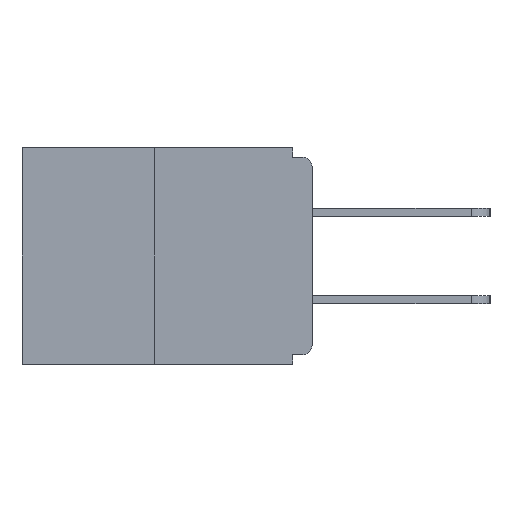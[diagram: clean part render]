
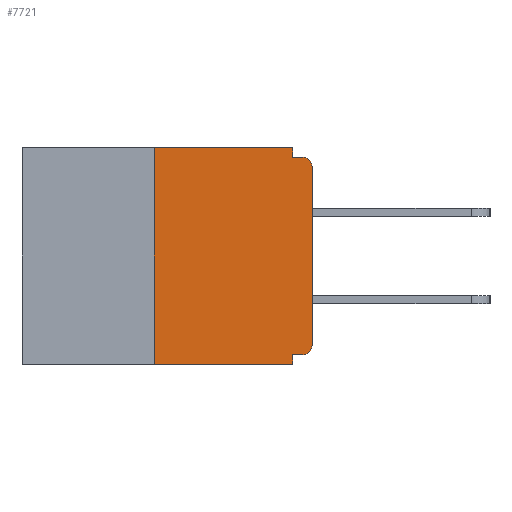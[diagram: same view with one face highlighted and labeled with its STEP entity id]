
A CAD part, left-side view. The second image highlights one B-rep face of the part: STEP entity #7721.
In plain terms, the highlighted planar face has unit normal (-1, 0, 0).
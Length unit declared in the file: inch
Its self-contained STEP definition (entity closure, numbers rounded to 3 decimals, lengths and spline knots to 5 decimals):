
#87 = CARTESIAN_POINT ( 'NONE',  ( 0., 0., -0.328 ) ) ;
#189 = CARTESIAN_POINT ( 'NONE',  ( 0., 0., 0. ) ) ;
#218 = ORIENTED_EDGE ( 'NONE', *, *, #12338, .T. ) ;
#695 = DIRECTION ( 'NONE',  ( 1., 0., 0. ) ) ;
#977 = CARTESIAN_POINT ( 'NONE',  ( 0., 0.031, 0. ) ) ;
#1492 = AXIS2_PLACEMENT_3D ( 'NONE', #21524, #695, #2453 ) ;
#1851 = DIRECTION ( 'NONE',  ( 0., 0., -1. ) ) ;
#1972 = DIRECTION ( 'NONE',  ( 0., 0., -1. ) ) ;
#1976 = VECTOR ( 'NONE', #21056, 39.37008 ) ;
#2016 = CIRCLE ( 'NONE', #18868, 0.015 ) ;
#2453 = DIRECTION ( 'NONE',  ( 0., 0., -1. ) ) ;
#2522 = ORIENTED_EDGE ( 'NONE', *, *, #21135, .F. ) ;
#3196 = CARTESIAN_POINT ( 'NONE',  ( 0., 0., -0.03 ) ) ;
#3369 = CARTESIAN_POINT ( 'NONE',  ( 0., 0.25, -0.343 ) ) ;
#4028 = EDGE_CURVE ( 'NONE', #12439, #8589, #10432, .T. ) ;
#4132 = DIRECTION ( 'NONE',  ( 0., 1., 0. ) ) ;
#4145 = VECTOR ( 'NONE', #10643, 39.37008 ) ;
#4317 = LINE ( 'NONE', #5608, #10608 ) ;
#4392 = ORIENTED_EDGE ( 'NONE', *, *, #21631, .T. ) ;
#4713 = VECTOR ( 'NONE', #19308, 39.37008 ) ;
#4917 = CARTESIAN_POINT ( 'NONE',  ( 0., 0.031, -0.015 ) ) ;
#4936 = ORIENTED_EDGE ( 'NONE', *, *, #24566, .F. ) ;
#5274 = CARTESIAN_POINT ( 'NONE',  ( 0., 0.25, 0. ) ) ;
#5608 = CARTESIAN_POINT ( 'NONE',  ( 0., 0.46, -0.343 ) ) ;
#5776 = CARTESIAN_POINT ( 'NONE',  ( 0., 0.015, -0.328 ) ) ;
#5835 = LINE ( 'NONE', #24543, #6129 ) ;
#6129 = VECTOR ( 'NONE', #10863, 39.37008 ) ;
#6374 = ORIENTED_EDGE ( 'NONE', *, *, #9918, .T. ) ;
#6804 = CARTESIAN_POINT ( 'NONE',  ( 0., 0.031, -0.343 ) ) ;
#6998 = DIRECTION ( 'NONE',  ( -1., 0., 0. ) ) ;
#7721 = ADVANCED_FACE ( 'NONE', ( #10244 ), #21444, .F. ) ;
#7835 = EDGE_CURVE ( 'NONE', #17323, #21360, #9649, .T. ) ;
#8450 = CARTESIAN_POINT ( 'NONE',  ( 0., 0.015, -0.015 ) ) ;
#8589 = VERTEX_POINT ( 'NONE', #24589 ) ;
#8884 = VERTEX_POINT ( 'NONE', #5274 ) ;
#9649 = LINE ( 'NONE', #20256, #17403 ) ;
#9728 = VERTEX_POINT ( 'NONE', #977 ) ;
#9918 = EDGE_CURVE ( 'NONE', #16723, #21360, #11314, .T. ) ;
#10037 = LINE ( 'NONE', #12642, #1976 ) ;
#10227 = ORIENTED_EDGE ( 'NONE', *, *, #11829, .F. ) ;
#10244 = FACE_OUTER_BOUND ( 'NONE', #12458, .T. ) ;
#10353 = VERTEX_POINT ( 'NONE', #5776 ) ;
#10432 = LINE ( 'NONE', #6804, #4145 ) ;
#10608 = VECTOR ( 'NONE', #17289, 39.37008 ) ;
#10643 = DIRECTION ( 'NONE',  ( 0., 0., -1. ) ) ;
#10863 = DIRECTION ( 'NONE',  ( 0., -1., 0. ) ) ;
#11314 = CIRCLE ( 'NONE', #18311, 0.015 ) ;
#11829 = EDGE_CURVE ( 'NONE', #10353, #12439, #13964, .T. ) ;
#12338 = EDGE_CURVE ( 'NONE', #18425, #16723, #15742, .T. ) ;
#12439 = VERTEX_POINT ( 'NONE', #14061 ) ;
#12458 = EDGE_LOOP ( 'NONE', ( #4936, #2522, #4392, #22076, #10227, #15150, #218, #6374, #20806, #23086 ) ) ;
#12642 = CARTESIAN_POINT ( 'NONE',  ( 0., 0.25, 0. ) ) ;
#13340 = VECTOR ( 'NONE', #1851, 39.37008 ) ;
#13652 = EDGE_CURVE ( 'NONE', #10353, #18425, #2016, .T. ) ;
#13964 = LINE ( 'NONE', #87, #22417 ) ;
#14061 = CARTESIAN_POINT ( 'NONE',  ( 0., 0.031, -0.328 ) ) ;
#14726 = CARTESIAN_POINT ( 'NONE',  ( 0., 0., -0.313 ) ) ;
#15150 = ORIENTED_EDGE ( 'NONE', *, *, #13652, .T. ) ;
#15742 = LINE ( 'NONE', #189, #4713 ) ;
#16723 = VERTEX_POINT ( 'NONE', #3196 ) ;
#17142 = DIRECTION ( 'NONE',  ( -1., 0., 0. ) ) ;
#17289 = DIRECTION ( 'NONE',  ( 0., -1., 0. ) ) ;
#17323 = VERTEX_POINT ( 'NONE', #4917 ) ;
#17403 = VECTOR ( 'NONE', #24103, 39.37008 ) ;
#18311 = AXIS2_PLACEMENT_3D ( 'NONE', #21044, #17142, #1972 ) ;
#18425 = VERTEX_POINT ( 'NONE', #14726 ) ;
#18755 = LINE ( 'NONE', #21001, #13340 ) ;
#18868 = AXIS2_PLACEMENT_3D ( 'NONE', #22333, #6998, #20416 ) ;
#19308 = DIRECTION ( 'NONE',  ( 0., 0., 1. ) ) ;
#20233 = VERTEX_POINT ( 'NONE', #3369 ) ;
#20256 = CARTESIAN_POINT ( 'NONE',  ( 0., 0., -0.015 ) ) ;
#20416 = DIRECTION ( 'NONE',  ( 0., 0., -1. ) ) ;
#20806 = ORIENTED_EDGE ( 'NONE', *, *, #7835, .F. ) ;
#21001 = CARTESIAN_POINT ( 'NONE',  ( 0., 0.031, 0. ) ) ;
#21044 = CARTESIAN_POINT ( 'NONE',  ( 0., 0.015, -0.03 ) ) ;
#21056 = DIRECTION ( 'NONE',  ( 0., 0., 1. ) ) ;
#21135 = EDGE_CURVE ( 'NONE', #20233, #8884, #10037, .T. ) ;
#21360 = VERTEX_POINT ( 'NONE', #8450 ) ;
#21444 = PLANE ( 'NONE',  #1492 ) ;
#21524 = CARTESIAN_POINT ( 'NONE',  ( 0., 0.46, 0. ) ) ;
#21631 = EDGE_CURVE ( 'NONE', #20233, #8589, #4317, .T. ) ;
#22076 = ORIENTED_EDGE ( 'NONE', *, *, #4028, .F. ) ;
#22333 = CARTESIAN_POINT ( 'NONE',  ( 0., 0.015, -0.313 ) ) ;
#22417 = VECTOR ( 'NONE', #4132, 39.37008 ) ;
#23086 = ORIENTED_EDGE ( 'NONE', *, *, #23717, .F. ) ;
#23717 = EDGE_CURVE ( 'NONE', #9728, #17323, #18755, .T. ) ;
#24103 = DIRECTION ( 'NONE',  ( 0., -1., 0. ) ) ;
#24543 = CARTESIAN_POINT ( 'NONE',  ( 0., 0.46, 0. ) ) ;
#24566 = EDGE_CURVE ( 'NONE', #8884, #9728, #5835, .T. ) ;
#24589 = CARTESIAN_POINT ( 'NONE',  ( 0., 0.031, -0.343 ) ) ;
